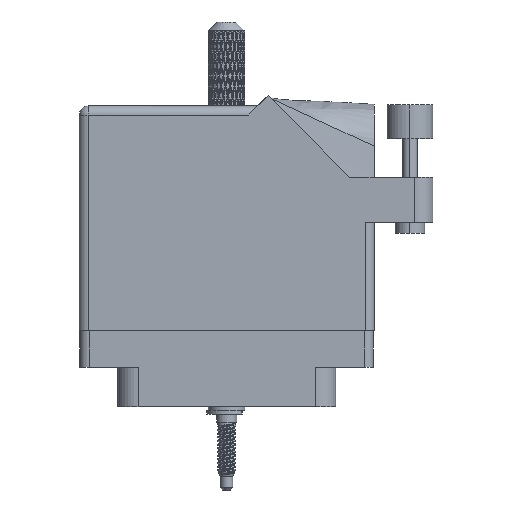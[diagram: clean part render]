
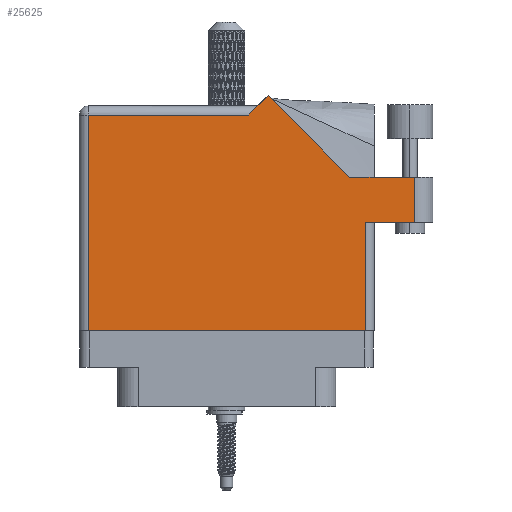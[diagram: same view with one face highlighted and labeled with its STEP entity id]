
A CAD part, front view. The second image highlights one B-rep face of the part: STEP entity #25625.
In plain terms, the highlighted face is planar.
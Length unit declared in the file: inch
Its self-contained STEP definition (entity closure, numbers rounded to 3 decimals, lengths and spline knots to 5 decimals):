
#3065 = DIRECTION ( 'NONE',  ( 0., 1., 0. ) ) ;
#3496 = LINE ( 'NONE', #39808, #58988 ) ;
#4242 = CARTESIAN_POINT ( 'NONE',  ( 0.943, 0.637, 0.455 ) ) ;
#6681 = CARTESIAN_POINT ( 'NONE',  ( -0.943, -0.1, 0.455 ) ) ;
#9745 = LINE ( 'NONE', #31191, #43038 ) ;
#10283 = ORIENTED_EDGE ( 'NONE', *, *, #98692, .T. ) ;
#10638 = DIRECTION ( 'NONE',  ( -1., 0., 0. ) ) ;
#11162 = LINE ( 'NONE', #15329, #99733 ) ;
#12243 = VERTEX_POINT ( 'NONE', #12967 ) ;
#12435 = VECTOR ( 'NONE', #3065, 39.37008 ) ;
#12967 = CARTESIAN_POINT ( 'NONE',  ( 0.15, 1.368, 0.455 ) ) ;
#15329 = CARTESIAN_POINT ( 'NONE',  ( -1.005, 1.368, 0.455 ) ) ;
#16604 = ORIENTED_EDGE ( 'NONE', *, *, #59816, .T. ) ;
#18934 = EDGE_CURVE ( 'NONE', #33164, #86781, #37294, .T. ) ;
#23617 = CARTESIAN_POINT ( 'NONE',  ( -1.005, -0.1, 0.455 ) ) ;
#25210 = CARTESIAN_POINT ( 'NONE',  ( 0.212, 1.43, 0.455 ) ) ;
#25625 = ADVANCED_FACE ( 'NONE', ( #69994 ), #62313, .F. ) ;
#26094 = CARTESIAN_POINT ( 'NONE',  ( 1.405, 0.944, 0.455 ) ) ;
#26301 = CARTESIAN_POINT ( 'NONE',  ( -0.943, -0.1, 0.455 ) ) ;
#26527 = CARTESIAN_POINT ( 'NONE',  ( 1.28, 0.944, 0.455 ) ) ;
#28239 = LINE ( 'NONE', #62617, #90905 ) ;
#31191 = CARTESIAN_POINT ( 'NONE',  ( 0.943, 0.637, 0.455 ) ) ;
#31396 = EDGE_LOOP ( 'NONE', ( #35407, #54393, #61469, #16604, #10283, #51086, #69977, #81951, #36178 ) ) ;
#32905 = VERTEX_POINT ( 'NONE', #81117 ) ;
#33164 = VERTEX_POINT ( 'NONE', #95146 ) ;
#35407 = ORIENTED_EDGE ( 'NONE', *, *, #92371, .T. ) ;
#36120 = EDGE_CURVE ( 'NONE', #86781, #32905, #39093, .T. ) ;
#36178 = ORIENTED_EDGE ( 'NONE', *, *, #50652, .T. ) ;
#36701 = VERTEX_POINT ( 'NONE', #86705 ) ;
#37294 = LINE ( 'NONE', #26301, #97502 ) ;
#38881 = CARTESIAN_POINT ( 'NONE',  ( -1.005, 1.43, 0.455 ) ) ;
#39093 = LINE ( 'NONE', #23617, #69908 ) ;
#39808 = CARTESIAN_POINT ( 'NONE',  ( 0.83942, 0.944, 0.455 ) ) ;
#43038 = VECTOR ( 'NONE', #70679, 39.37008 ) ;
#47704 = EDGE_CURVE ( 'NONE', #101845, #87140, #72762, .T. ) ;
#50522 = VERTEX_POINT ( 'NONE', #92992 ) ;
#50652 = EDGE_CURVE ( 'NONE', #32905, #99980, #9745, .T. ) ;
#51086 = ORIENTED_EDGE ( 'NONE', *, *, #101123, .T. ) ;
#52281 = VECTOR ( 'NONE', #87711, 39.37008 ) ;
#54215 = DIRECTION ( 'NONE',  ( -1., 0., 0. ) ) ;
#54393 = ORIENTED_EDGE ( 'NONE', *, *, #47704, .T. ) ;
#57284 = EDGE_CURVE ( 'NONE', #87140, #36701, #81384, .T. ) ;
#58988 = VECTOR ( 'NONE', #93421, 39.37008 ) ;
#59816 = EDGE_CURVE ( 'NONE', #36701, #50522, #3496, .T. ) ;
#61469 = ORIENTED_EDGE ( 'NONE', *, *, #57284, .T. ) ;
#62313 = PLANE ( 'NONE',  #85723 ) ;
#62617 = CARTESIAN_POINT ( 'NONE',  ( 1.005, 0.637, 0.455 ) ) ;
#69908 = VECTOR ( 'NONE', #101668, 39.37008 ) ;
#69977 = ORIENTED_EDGE ( 'NONE', *, *, #18934, .T. ) ;
#69994 = FACE_OUTER_BOUND ( 'NONE', #31396, .T. ) ;
#70679 = DIRECTION ( 'NONE',  ( 0., 1., 0. ) ) ;
#72762 = LINE ( 'NONE', #26527, #12435 ) ;
#79043 = DIRECTION ( 'NONE',  ( 1., 0., 0. ) ) ;
#81117 = CARTESIAN_POINT ( 'NONE',  ( 0.943, -0.1, 0.455 ) ) ;
#81265 = DIRECTION ( 'NONE',  ( 0., -1., 0. ) ) ;
#81384 = LINE ( 'NONE', #26094, #87459 ) ;
#81951 = ORIENTED_EDGE ( 'NONE', *, *, #36120, .T. ) ;
#85723 = AXIS2_PLACEMENT_3D ( 'NONE', #38881, #93840, #101777 ) ;
#86705 = CARTESIAN_POINT ( 'NONE',  ( 0.83942, 0.944, 0.455 ) ) ;
#86781 = VERTEX_POINT ( 'NONE', #6681 ) ;
#87140 = VERTEX_POINT ( 'NONE', #94843 ) ;
#87459 = VECTOR ( 'NONE', #10638, 39.37008 ) ;
#87711 = DIRECTION ( 'NONE',  ( -0.707, -0.707, 0. ) ) ;
#87742 = LINE ( 'NONE', #25210, #52281 ) ;
#90905 = VECTOR ( 'NONE', #79043, 39.37008 ) ;
#92371 = EDGE_CURVE ( 'NONE', #99980, #101845, #28239, .T. ) ;
#92992 = CARTESIAN_POINT ( 'NONE',  ( 0.28271, 1.50071, 0.455 ) ) ;
#93421 = DIRECTION ( 'NONE',  ( -0.707, 0.707, 0. ) ) ;
#93840 = DIRECTION ( 'NONE',  ( 0., 0., -1. ) ) ;
#94843 = CARTESIAN_POINT ( 'NONE',  ( 1.28, 0.944, 0.455 ) ) ;
#95146 = CARTESIAN_POINT ( 'NONE',  ( -0.943, 1.368, 0.455 ) ) ;
#97502 = VECTOR ( 'NONE', #81265, 39.37008 ) ;
#98692 = EDGE_CURVE ( 'NONE', #50522, #12243, #87742, .T. ) ;
#99733 = VECTOR ( 'NONE', #54215, 39.37008 ) ;
#99980 = VERTEX_POINT ( 'NONE', #4242 ) ;
#101123 = EDGE_CURVE ( 'NONE', #12243, #33164, #11162, .T. ) ;
#101230 = CARTESIAN_POINT ( 'NONE',  ( 1.28, 0.637, 0.455 ) ) ;
#101668 = DIRECTION ( 'NONE',  ( 1., 0., 0. ) ) ;
#101777 = DIRECTION ( 'NONE',  ( -1., 0., 0. ) ) ;
#101845 = VERTEX_POINT ( 'NONE', #101230 ) ;
